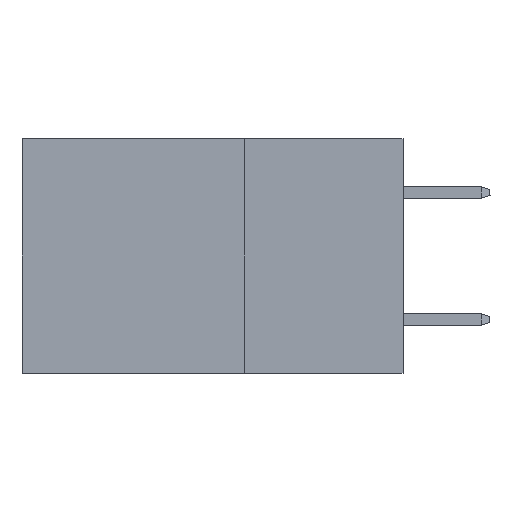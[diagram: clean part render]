
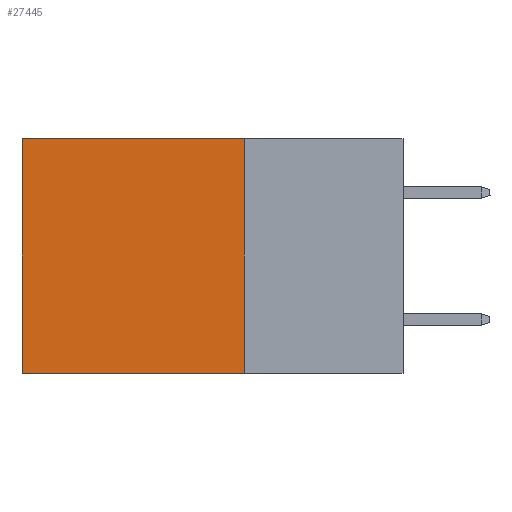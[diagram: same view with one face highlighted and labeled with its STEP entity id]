
A CAD part, left-side view. The second image highlights one B-rep face of the part: STEP entity #27445.
In plain terms, the highlighted planar face has unit normal (-1, 0, 0).
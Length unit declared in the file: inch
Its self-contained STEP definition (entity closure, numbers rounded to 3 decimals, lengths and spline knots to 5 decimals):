
#570 = EDGE_CURVE ( 'NONE', #5317, #32019, #26062, .T. ) ;
#1702 = LINE ( 'NONE', #11681, #21850 ) ;
#2037 = CARTESIAN_POINT ( 'NONE',  ( 0.2875, 0.25, 0. ) ) ;
#2323 = CARTESIAN_POINT ( 'NONE',  ( 0.2875, 0.25, -0.37 ) ) ;
#3094 = EDGE_CURVE ( 'NONE', #32019, #12941, #8456, .T. ) ;
#3668 = DIRECTION ( 'NONE',  ( 0., 1., 0. ) ) ;
#4714 = FACE_OUTER_BOUND ( 'NONE', #22353, .T. ) ;
#4868 = EDGE_CURVE ( 'NONE', #21830, #12941, #1702, .T. ) ;
#5317 = VERTEX_POINT ( 'NONE', #14561 ) ;
#6632 = LINE ( 'NONE', #2037, #16475 ) ;
#6789 = DIRECTION ( 'NONE',  ( 0., 0., -1. ) ) ;
#8456 = LINE ( 'NONE', #21377, #21828 ) ;
#11138 = ORIENTED_EDGE ( 'NONE', *, *, #4868, .F. ) ;
#11681 = CARTESIAN_POINT ( 'NONE',  ( 0.2875, 0.25, -0.37 ) ) ;
#11990 = AXIS2_PLACEMENT_3D ( 'NONE', #21755, #14527, #14692 ) ;
#12941 = VERTEX_POINT ( 'NONE', #25972 ) ;
#14527 = DIRECTION ( 'NONE',  ( 1., 0., 0. ) ) ;
#14561 = CARTESIAN_POINT ( 'NONE',  ( 0.2875, 0.25, 0. ) ) ;
#14692 = DIRECTION ( 'NONE',  ( 0., 0., -1. ) ) ;
#16475 = VECTOR ( 'NONE', #6789, 39.37008 ) ;
#17278 = CARTESIAN_POINT ( 'NONE',  ( 0.2875, 0.6, 0. ) ) ;
#19285 = PLANE ( 'NONE',  #11990 ) ;
#20092 = EDGE_CURVE ( 'NONE', #5317, #21830, #6632, .T. ) ;
#21377 = CARTESIAN_POINT ( 'NONE',  ( 0.2875, 0.6, 0. ) ) ;
#21675 = DIRECTION ( 'NONE',  ( 0., 1., 0. ) ) ;
#21755 = CARTESIAN_POINT ( 'NONE',  ( 0.2875, 0.25, 0. ) ) ;
#21828 = VECTOR ( 'NONE', #31330, 39.37008 ) ;
#21830 = VERTEX_POINT ( 'NONE', #2323 ) ;
#21850 = VECTOR ( 'NONE', #21675, 39.37008 ) ;
#22353 = EDGE_LOOP ( 'NONE', ( #25843, #11138, #24828, #25250 ) ) ;
#24828 = ORIENTED_EDGE ( 'NONE', *, *, #20092, .F. ) ;
#25250 = ORIENTED_EDGE ( 'NONE', *, *, #570, .T. ) ;
#25843 = ORIENTED_EDGE ( 'NONE', *, *, #3094, .T. ) ;
#25972 = CARTESIAN_POINT ( 'NONE',  ( 0.2875, 0.6, -0.37 ) ) ;
#26062 = LINE ( 'NONE', #26219, #32283 ) ;
#26219 = CARTESIAN_POINT ( 'NONE',  ( 0.2875, 0.25, 0. ) ) ;
#27445 = ADVANCED_FACE ( 'NONE', ( #4714 ), #19285, .F. ) ;
#31330 = DIRECTION ( 'NONE',  ( 0., 0., -1. ) ) ;
#32019 = VERTEX_POINT ( 'NONE', #17278 ) ;
#32283 = VECTOR ( 'NONE', #3668, 39.37008 ) ;
